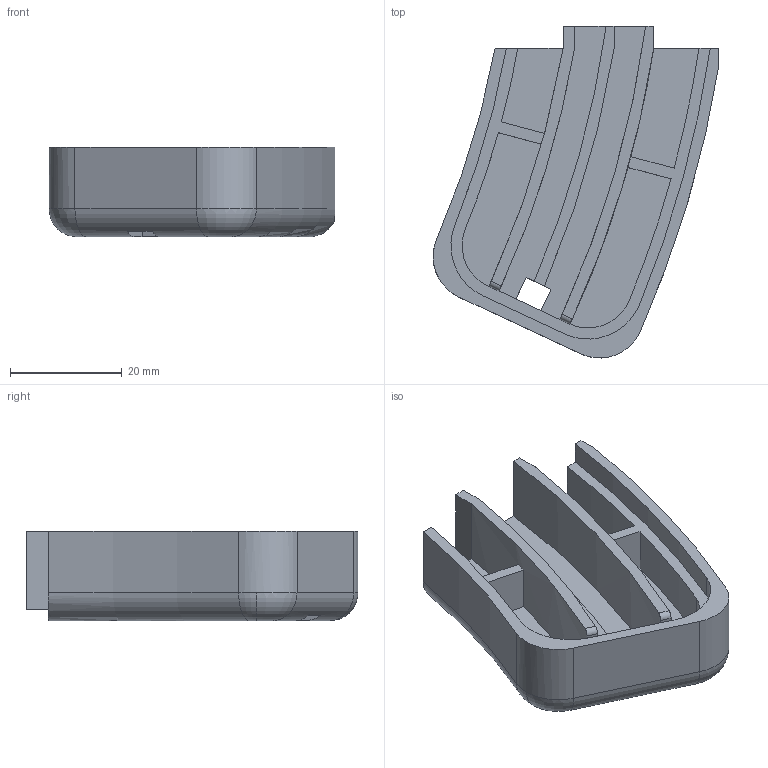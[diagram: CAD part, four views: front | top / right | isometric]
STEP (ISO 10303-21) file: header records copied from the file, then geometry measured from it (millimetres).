
FILE_DESCRIPTION (( 'STEP AP214' ), '1' );
FILE_NAME ('left_small.STEP', '2013-07-01T00:26:06', ( '' ), ( '' ), 'SwSTEP 2.0', 'SolidWorks 2013', '' );
FILE_SCHEMA (( 'AUTOMOTIVE_DESIGN' ));
Length unit declared in the file: millimetre
Products named in the file (1): left_small
Bounding box: 51.13 x 59.38 x 16 mm (x, y, z)
Volume: 15923.6 mm3; surface area: 10740.1 mm2
Topology: 1 solids, 1 shells, 63 faces, 180 edges, 117 vertices
Faces by surface type: plane 35, cylinder 23, torus 5
Entity records: 2157 total; most frequent: CARTESIAN_POINT 434, ORIENTED_EDGE 360, DIRECTION 359, EDGE_CURVE 180, AXIS2_PLACEMENT_3D 122, VERTEX_POINT 117, LINE 115, VECTOR 115
